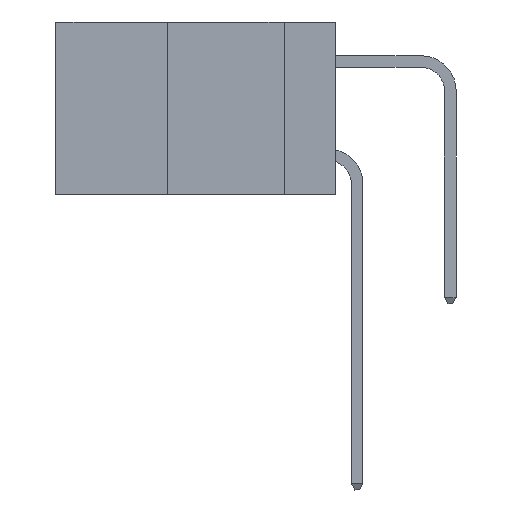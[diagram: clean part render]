
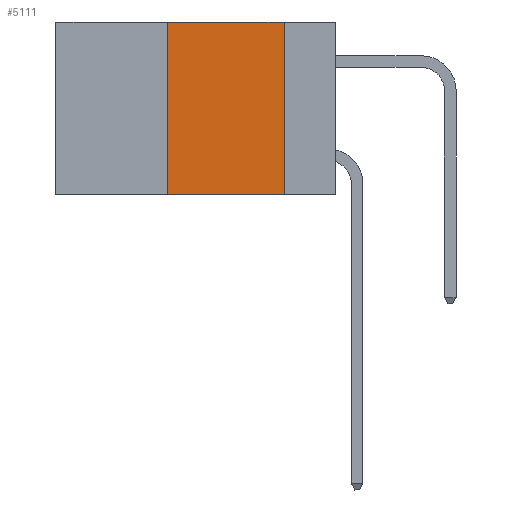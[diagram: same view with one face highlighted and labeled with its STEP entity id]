
A CAD part, left-side view. The second image highlights one B-rep face of the part: STEP entity #5111.
In plain terms, the highlighted planar face has unit normal (-1, 0, 0).
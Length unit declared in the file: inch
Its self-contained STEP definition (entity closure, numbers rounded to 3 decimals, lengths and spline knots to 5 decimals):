
#178 = DIRECTION ( 'NONE',  ( 0., -1., 0. ) ) ;
#905 = EDGE_CURVE ( 'NONE', #15002, #23087, #1470, .T. ) ;
#1470 = LINE ( 'NONE', #18480, #20495 ) ;
#1694 = CARTESIAN_POINT ( 'NONE',  ( 0., 0.36, 0. ) ) ;
#1743 = VECTOR ( 'NONE', #2573, 39.37008 ) ;
#2385 = ORIENTED_EDGE ( 'NONE', *, *, #20237, .F. ) ;
#2573 = DIRECTION ( 'NONE',  ( 0., -1., 0. ) ) ;
#4528 = FACE_OUTER_BOUND ( 'NONE', #15080, .T. ) ;
#4991 = AXIS2_PLACEMENT_3D ( 'NONE', #14223, #19915, #8891 ) ;
#5111 = ADVANCED_FACE ( 'NONE', ( #4528 ), #7071, .F. ) ;
#6368 = CARTESIAN_POINT ( 'NONE',  ( 0., 0.6, 0. ) ) ;
#6777 = VERTEX_POINT ( 'NONE', #15268 ) ;
#7071 = PLANE ( 'NONE',  #4991 ) ;
#7750 = LINE ( 'NONE', #1694, #12545 ) ;
#7783 = ORIENTED_EDGE ( 'NONE', *, *, #23430, .F. ) ;
#7899 = ORIENTED_EDGE ( 'NONE', *, *, #905, .F. ) ;
#8372 = LINE ( 'NONE', #22180, #13190 ) ;
#8891 = DIRECTION ( 'NONE',  ( 0., 0., -1. ) ) ;
#11101 = CARTESIAN_POINT ( 'NONE',  ( 0., 0.11, 0. ) ) ;
#11553 = LINE ( 'NONE', #6368, #1743 ) ;
#12545 = VECTOR ( 'NONE', #12700, 39.37008 ) ;
#12700 = DIRECTION ( 'NONE',  ( 0., 0., 1. ) ) ;
#13190 = VECTOR ( 'NONE', #178, 39.37008 ) ;
#14223 = CARTESIAN_POINT ( 'NONE',  ( 0., 0.6, 0. ) ) ;
#15002 = VERTEX_POINT ( 'NONE', #11101 ) ;
#15080 = EDGE_LOOP ( 'NONE', ( #7899, #2385, #7783, #20011 ) ) ;
#15268 = CARTESIAN_POINT ( 'NONE',  ( 0., 0.36, 0. ) ) ;
#15405 = CARTESIAN_POINT ( 'NONE',  ( 0., 0.11, -0.37 ) ) ;
#15406 = VERTEX_POINT ( 'NONE', #22777 ) ;
#17997 = DIRECTION ( 'NONE',  ( 0., 0., -1. ) ) ;
#18480 = CARTESIAN_POINT ( 'NONE',  ( 0., 0.11, 0. ) ) ;
#19915 = DIRECTION ( 'NONE',  ( 1., 0., 0. ) ) ;
#20011 = ORIENTED_EDGE ( 'NONE', *, *, #22264, .T. ) ;
#20237 = EDGE_CURVE ( 'NONE', #6777, #15002, #11553, .T. ) ;
#20495 = VECTOR ( 'NONE', #17997, 39.37008 ) ;
#22180 = CARTESIAN_POINT ( 'NONE',  ( 0., 0.6, -0.37 ) ) ;
#22264 = EDGE_CURVE ( 'NONE', #15406, #23087, #8372, .T. ) ;
#22777 = CARTESIAN_POINT ( 'NONE',  ( 0., 0.36, -0.37 ) ) ;
#23087 = VERTEX_POINT ( 'NONE', #15405 ) ;
#23430 = EDGE_CURVE ( 'NONE', #15406, #6777, #7750, .T. ) ;
